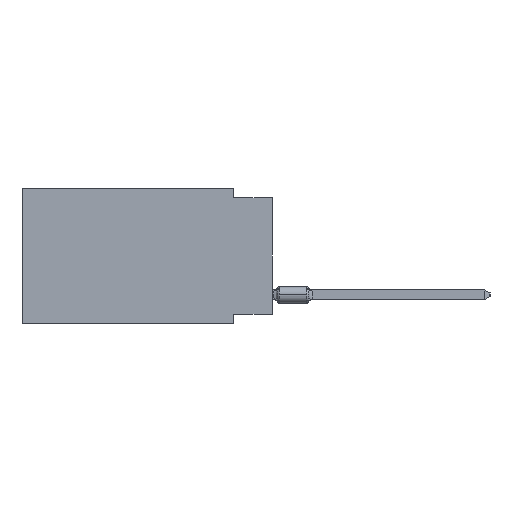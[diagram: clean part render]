
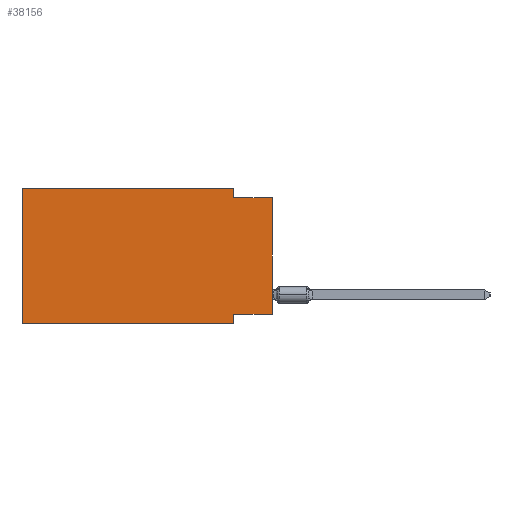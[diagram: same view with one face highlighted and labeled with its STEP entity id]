
A CAD part, left-side view. The second image highlights one B-rep face of the part: STEP entity #38156.
In plain terms, the highlighted planar face has unit normal (-1, 0, 0).
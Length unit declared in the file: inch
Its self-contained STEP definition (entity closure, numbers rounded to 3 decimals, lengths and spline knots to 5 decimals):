
#237 = EDGE_CURVE ( 'NONE', #31620, #49770, #1111, .T. ) ;
#1111 = LINE ( 'NONE', #13740, #51294 ) ;
#1336 = ORIENTED_EDGE ( 'NONE', *, *, #55567, .F. ) ;
#3550 = DIRECTION ( 'NONE',  ( 0., 0., 1. ) ) ;
#3623 = CARTESIAN_POINT ( 'NONE',  ( 0., 0.645, 0. ) ) ;
#4493 = DIRECTION ( 'NONE',  ( 0., 0., 1. ) ) ;
#4883 = LINE ( 'NONE', #44524, #8540 ) ;
#5901 = CARTESIAN_POINT ( 'NONE',  ( 0., 0.645, 0. ) ) ;
#6180 = CARTESIAN_POINT ( 'NONE',  ( 0., 0.1, -0.35 ) ) ;
#6609 = ORIENTED_EDGE ( 'NONE', *, *, #31376, .T. ) ;
#7430 = EDGE_CURVE ( 'NONE', #53206, #40891, #54156, .T. ) ;
#8540 = VECTOR ( 'NONE', #26705, 39.37008 ) ;
#9634 = LINE ( 'NONE', #5901, #46144 ) ;
#10854 = VERTEX_POINT ( 'NONE', #14047 ) ;
#11657 = PLANE ( 'NONE',  #32803 ) ;
#12209 = EDGE_CURVE ( 'NONE', #49369, #40891, #13844, .T. ) ;
#12526 = LINE ( 'NONE', #52750, #30479 ) ;
#13740 = CARTESIAN_POINT ( 'NONE',  ( 0., 0., -0.025 ) ) ;
#13844 = LINE ( 'NONE', #21604, #15876 ) ;
#14047 = CARTESIAN_POINT ( 'NONE',  ( 0., 0., -0.325 ) ) ;
#15876 = VECTOR ( 'NONE', #44296, 39.37008 ) ;
#16638 = CARTESIAN_POINT ( 'NONE',  ( 0., 0.645, -0.35 ) ) ;
#18294 = CARTESIAN_POINT ( 'NONE',  ( 0., 0.1, 0. ) ) ;
#18805 = CARTESIAN_POINT ( 'NONE',  ( 0., 0.645, 0. ) ) ;
#21173 = CARTESIAN_POINT ( 'NONE',  ( 0., 0., -0.025 ) ) ;
#21604 = CARTESIAN_POINT ( 'NONE',  ( 0., 0.645, -0.35 ) ) ;
#25751 = CARTESIAN_POINT ( 'NONE',  ( 0., 0.1, 0. ) ) ;
#26705 = DIRECTION ( 'NONE',  ( 0., 1., 0. ) ) ;
#27477 = ORIENTED_EDGE ( 'NONE', *, *, #237, .F. ) ;
#27523 = ORIENTED_EDGE ( 'NONE', *, *, #12209, .T. ) ;
#27705 = CARTESIAN_POINT ( 'NONE',  ( 0., 0.1, -0.35 ) ) ;
#30284 = VECTOR ( 'NONE', #41225, 39.37008 ) ;
#30479 = VECTOR ( 'NONE', #4493, 39.37008 ) ;
#30964 = ORIENTED_EDGE ( 'NONE', *, *, #45301, .F. ) ;
#31279 = VERTEX_POINT ( 'NONE', #18294 ) ;
#31376 = EDGE_CURVE ( 'NONE', #10854, #49770, #55833, .T. ) ;
#31620 = VERTEX_POINT ( 'NONE', #39699 ) ;
#31927 = EDGE_CURVE ( 'NONE', #10854, #53206, #4883, .T. ) ;
#32287 = EDGE_LOOP ( 'NONE', ( #6609, #27477, #1336, #30964, #35021, #27523, #47833, #34974 ) ) ;
#32325 = CARTESIAN_POINT ( 'NONE',  ( 0., 0.1, -0.325 ) ) ;
#32803 = AXIS2_PLACEMENT_3D ( 'NONE', #3623, #34063, #46425 ) ;
#34063 = DIRECTION ( 'NONE',  ( 1., 0., 0. ) ) ;
#34974 = ORIENTED_EDGE ( 'NONE', *, *, #31927, .F. ) ;
#35021 = ORIENTED_EDGE ( 'NONE', *, *, #45139, .F. ) ;
#36714 = DIRECTION ( 'NONE',  ( 0., -1., 0. ) ) ;
#38156 = ADVANCED_FACE ( 'NONE', ( #42966 ), #11657, .F. ) ;
#38958 = DIRECTION ( 'NONE',  ( 0., 0., -1. ) ) ;
#39699 = CARTESIAN_POINT ( 'NONE',  ( 0., 0.1, -0.025 ) ) ;
#40099 = DIRECTION ( 'NONE',  ( 0., -1., 0. ) ) ;
#40826 = VERTEX_POINT ( 'NONE', #18805 ) ;
#40891 = VERTEX_POINT ( 'NONE', #27705 ) ;
#41225 = DIRECTION ( 'NONE',  ( 0., 0., -1. ) ) ;
#42714 = LINE ( 'NONE', #25751, #56021 ) ;
#42966 = FACE_OUTER_BOUND ( 'NONE', #32287, .T. ) ;
#44296 = DIRECTION ( 'NONE',  ( 0., -1., 0. ) ) ;
#44524 = CARTESIAN_POINT ( 'NONE',  ( 0., 0., -0.325 ) ) ;
#45139 = EDGE_CURVE ( 'NONE', #49369, #40826, #12526, .T. ) ;
#45301 = EDGE_CURVE ( 'NONE', #40826, #31279, #9634, .T. ) ;
#46144 = VECTOR ( 'NONE', #40099, 39.37008 ) ;
#46425 = DIRECTION ( 'NONE',  ( 0., 0., -1. ) ) ;
#47833 = ORIENTED_EDGE ( 'NONE', *, *, #7430, .F. ) ;
#49369 = VERTEX_POINT ( 'NONE', #16638 ) ;
#49770 = VERTEX_POINT ( 'NONE', #21173 ) ;
#49806 = VECTOR ( 'NONE', #3550, 39.37008 ) ;
#51294 = VECTOR ( 'NONE', #36714, 39.37008 ) ;
#52750 = CARTESIAN_POINT ( 'NONE',  ( 0., 0.645, 0. ) ) ;
#53206 = VERTEX_POINT ( 'NONE', #32325 ) ;
#54156 = LINE ( 'NONE', #6180, #30284 ) ;
#55544 = CARTESIAN_POINT ( 'NONE',  ( 0., 0., 0. ) ) ;
#55567 = EDGE_CURVE ( 'NONE', #31279, #31620, #42714, .T. ) ;
#55833 = LINE ( 'NONE', #55544, #49806 ) ;
#56021 = VECTOR ( 'NONE', #38958, 39.37008 ) ;
